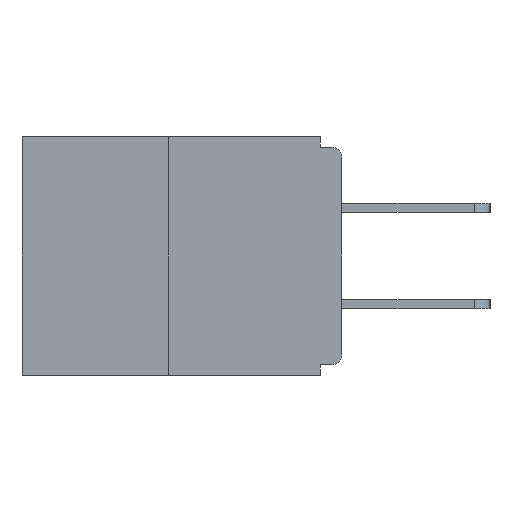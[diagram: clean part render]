
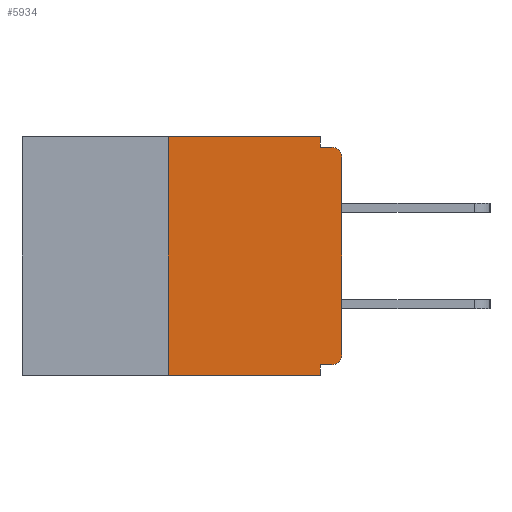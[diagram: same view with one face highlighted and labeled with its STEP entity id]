
A CAD part, left-side view. The second image highlights one B-rep face of the part: STEP entity #5934.
In plain terms, the highlighted planar face has unit normal (-1, 0, 0).
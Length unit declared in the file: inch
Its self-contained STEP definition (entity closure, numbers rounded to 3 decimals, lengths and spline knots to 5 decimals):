
#132 = DIRECTION ( 'NONE',  ( 0., 0., -1. ) ) ;
#190 = CARTESIAN_POINT ( 'NONE',  ( 0., 0., 0. ) ) ;
#239 = EDGE_CURVE ( 'NONE', #1979, #10412, #9212, .T. ) ;
#277 = CIRCLE ( 'NONE', #12965, 0.015 ) ;
#351 = LINE ( 'NONE', #190, #12228 ) ;
#465 = VERTEX_POINT ( 'NONE', #10991 ) ;
#503 = VECTOR ( 'NONE', #12731, 39.37008 ) ;
#1390 = EDGE_CURVE ( 'NONE', #13422, #9604, #10014, .T. ) ;
#1501 = EDGE_CURVE ( 'NONE', #1979, #5467, #277, .T. ) ;
#1723 = ORIENTED_EDGE ( 'NONE', *, *, #8643, .F. ) ;
#1737 = CIRCLE ( 'NONE', #6145, 0.015 ) ;
#1906 = ORIENTED_EDGE ( 'NONE', *, *, #1390, .F. ) ;
#1979 = VERTEX_POINT ( 'NONE', #12279 ) ;
#2039 = VERTEX_POINT ( 'NONE', #5017 ) ;
#2090 = CARTESIAN_POINT ( 'NONE',  ( 0., 0.46, 0. ) ) ;
#2095 = AXIS2_PLACEMENT_3D ( 'NONE', #10993, #8864, #9983 ) ;
#2115 = VECTOR ( 'NONE', #7213, 39.37008 ) ;
#2295 = FACE_OUTER_BOUND ( 'NONE', #10476, .T. ) ;
#2502 = VECTOR ( 'NONE', #12808, 39.37008 ) ;
#2806 = EDGE_CURVE ( 'NONE', #10412, #465, #10972, .T. ) ;
#2853 = EDGE_CURVE ( 'NONE', #13422, #465, #7992, .T. ) ;
#3203 = CARTESIAN_POINT ( 'NONE',  ( 0., 0.46, -0.343 ) ) ;
#3379 = VERTEX_POINT ( 'NONE', #6061 ) ;
#3606 = CARTESIAN_POINT ( 'NONE',  ( 0., 0.25, -0.343 ) ) ;
#3943 = CARTESIAN_POINT ( 'NONE',  ( 0., 0., -0.313 ) ) ;
#4221 = CARTESIAN_POINT ( 'NONE',  ( 0., 0.015, -0.313 ) ) ;
#4302 = VECTOR ( 'NONE', #7409, 39.37008 ) ;
#4306 = CARTESIAN_POINT ( 'NONE',  ( 0., 0., -0.015 ) ) ;
#4705 = PLANE ( 'NONE',  #2095 ) ;
#5017 = CARTESIAN_POINT ( 'NONE',  ( 0., 0.031, 0. ) ) ;
#5284 = DIRECTION ( 'NONE',  ( 0., 0., -1. ) ) ;
#5294 = LINE ( 'NONE', #13531, #2115 ) ;
#5351 = CARTESIAN_POINT ( 'NONE',  ( 0., 0., -0.328 ) ) ;
#5467 = VERTEX_POINT ( 'NONE', #3943 ) ;
#5934 = ADVANCED_FACE ( 'NONE', ( #2295 ), #4705, .F. ) ;
#5998 = ORIENTED_EDGE ( 'NONE', *, *, #8742, .T. ) ;
#6061 = CARTESIAN_POINT ( 'NONE',  ( 0., 0., -0.03 ) ) ;
#6145 = AXIS2_PLACEMENT_3D ( 'NONE', #12954, #6568, #132 ) ;
#6536 = EDGE_CURVE ( 'NONE', #2039, #9398, #5294, .T. ) ;
#6568 = DIRECTION ( 'NONE',  ( -1., 0., 0. ) ) ;
#6682 = CARTESIAN_POINT ( 'NONE',  ( 0., 0.25, 0. ) ) ;
#6794 = EDGE_CURVE ( 'NONE', #9604, #2039, #7125, .T. ) ;
#7032 = VERTEX_POINT ( 'NONE', #13757 ) ;
#7125 = LINE ( 'NONE', #2090, #8117 ) ;
#7213 = DIRECTION ( 'NONE',  ( 0., 0., -1. ) ) ;
#7409 = DIRECTION ( 'NONE',  ( 0., 0., -1. ) ) ;
#7616 = DIRECTION ( 'NONE',  ( 0., -1., 0. ) ) ;
#7992 = LINE ( 'NONE', #3203, #10641 ) ;
#8104 = ORIENTED_EDGE ( 'NONE', *, *, #6536, .F. ) ;
#8117 = VECTOR ( 'NONE', #10679, 39.37008 ) ;
#8571 = ORIENTED_EDGE ( 'NONE', *, *, #1501, .T. ) ;
#8643 = EDGE_CURVE ( 'NONE', #9398, #7032, #12546, .T. ) ;
#8742 = EDGE_CURVE ( 'NONE', #5467, #3379, #351, .T. ) ;
#8864 = DIRECTION ( 'NONE',  ( 1., 0., 0. ) ) ;
#8920 = ORIENTED_EDGE ( 'NONE', *, *, #239, .F. ) ;
#9212 = LINE ( 'NONE', #5351, #2502 ) ;
#9303 = CARTESIAN_POINT ( 'NONE',  ( 0., 0.031, -0.015 ) ) ;
#9398 = VERTEX_POINT ( 'NONE', #9303 ) ;
#9604 = VERTEX_POINT ( 'NONE', #6682 ) ;
#9808 = ORIENTED_EDGE ( 'NONE', *, *, #6794, .F. ) ;
#9911 = ORIENTED_EDGE ( 'NONE', *, *, #10574, .T. ) ;
#9983 = DIRECTION ( 'NONE',  ( 0., 0., -1. ) ) ;
#9998 = ORIENTED_EDGE ( 'NONE', *, *, #2853, .T. ) ;
#10014 = LINE ( 'NONE', #12691, #10335 ) ;
#10335 = VECTOR ( 'NONE', #12734, 39.37008 ) ;
#10395 = CARTESIAN_POINT ( 'NONE',  ( 0., 0.031, -0.328 ) ) ;
#10412 = VERTEX_POINT ( 'NONE', #10395 ) ;
#10476 = EDGE_LOOP ( 'NONE', ( #9808, #1906, #9998, #13439, #8920, #8571, #5998, #9911, #1723, #8104 ) ) ;
#10574 = EDGE_CURVE ( 'NONE', #3379, #7032, #1737, .T. ) ;
#10641 = VECTOR ( 'NONE', #7616, 39.37008 ) ;
#10679 = DIRECTION ( 'NONE',  ( 0., -1., 0. ) ) ;
#10964 = DIRECTION ( 'NONE',  ( 0., 0., 1. ) ) ;
#10972 = LINE ( 'NONE', #12665, #4302 ) ;
#10991 = CARTESIAN_POINT ( 'NONE',  ( 0., 0.031, -0.343 ) ) ;
#10993 = CARTESIAN_POINT ( 'NONE',  ( 0., 0.46, 0. ) ) ;
#11655 = DIRECTION ( 'NONE',  ( -1., 0., 0. ) ) ;
#12228 = VECTOR ( 'NONE', #10964, 39.37008 ) ;
#12279 = CARTESIAN_POINT ( 'NONE',  ( 0., 0.015, -0.328 ) ) ;
#12546 = LINE ( 'NONE', #4306, #503 ) ;
#12665 = CARTESIAN_POINT ( 'NONE',  ( 0., 0.031, -0.343 ) ) ;
#12691 = CARTESIAN_POINT ( 'NONE',  ( 0., 0.25, 0. ) ) ;
#12731 = DIRECTION ( 'NONE',  ( 0., -1., 0. ) ) ;
#12734 = DIRECTION ( 'NONE',  ( 0., 0., 1. ) ) ;
#12808 = DIRECTION ( 'NONE',  ( 0., 1., 0. ) ) ;
#12954 = CARTESIAN_POINT ( 'NONE',  ( 0., 0.015, -0.03 ) ) ;
#12965 = AXIS2_PLACEMENT_3D ( 'NONE', #4221, #11655, #5284 ) ;
#13422 = VERTEX_POINT ( 'NONE', #3606 ) ;
#13439 = ORIENTED_EDGE ( 'NONE', *, *, #2806, .F. ) ;
#13531 = CARTESIAN_POINT ( 'NONE',  ( 0., 0.031, 0. ) ) ;
#13757 = CARTESIAN_POINT ( 'NONE',  ( 0., 0.015, -0.015 ) ) ;
